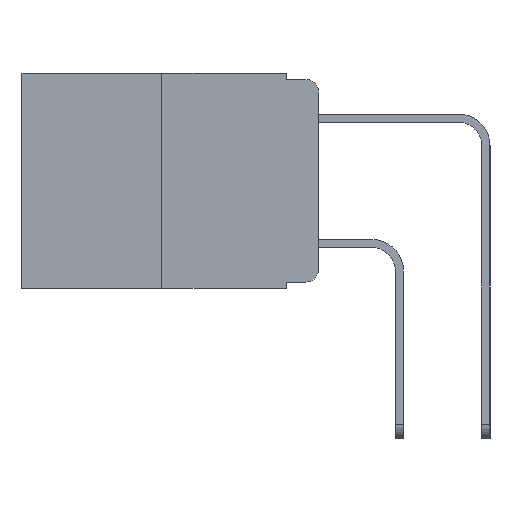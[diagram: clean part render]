
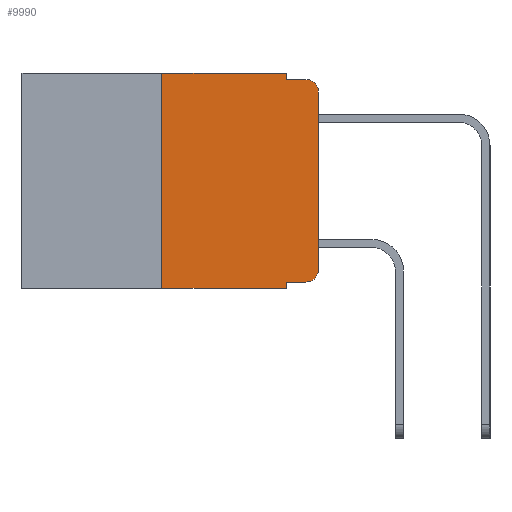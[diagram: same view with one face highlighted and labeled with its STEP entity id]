
A CAD part, left-side view. The second image highlights one B-rep face of the part: STEP entity #9990.
In plain terms, the highlighted planar face has unit normal (-1, 0, 0).
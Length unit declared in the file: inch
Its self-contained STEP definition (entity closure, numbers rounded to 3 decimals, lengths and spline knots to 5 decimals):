
#98 = ORIENTED_EDGE ( 'NONE', *, *, #17553, .T. ) ;
#219 = DIRECTION ( 'NONE',  ( 0., 0., -1. ) ) ;
#268 = VERTEX_POINT ( 'NONE', #16580 ) ;
#549 = CARTESIAN_POINT ( 'NONE',  ( 0., 0.25, -0.343 ) ) ;
#635 = ORIENTED_EDGE ( 'NONE', *, *, #16652, .T. ) ;
#702 = CARTESIAN_POINT ( 'NONE',  ( 0., 0.25, 0. ) ) ;
#779 = CARTESIAN_POINT ( 'NONE',  ( 0., 0.25, 0. ) ) ;
#1356 = DIRECTION ( 'NONE',  ( 0., 0., -1. ) ) ;
#1405 = DIRECTION ( 'NONE',  ( 1., 0., 0. ) ) ;
#2055 = DIRECTION ( 'NONE',  ( -1., 0., 0. ) ) ;
#2135 = ORIENTED_EDGE ( 'NONE', *, *, #11175, .F. ) ;
#2641 = CARTESIAN_POINT ( 'NONE',  ( 0., 0.473, -0.343 ) ) ;
#2648 = LINE ( 'NONE', #13618, #13686 ) ;
#3082 = ORIENTED_EDGE ( 'NONE', *, *, #9319, .T. ) ;
#3471 = DIRECTION ( 'NONE',  ( 0., -1., 0. ) ) ;
#3712 = VERTEX_POINT ( 'NONE', #13400 ) ;
#4144 = CARTESIAN_POINT ( 'NONE',  ( 0., 0.051, -0.343 ) ) ;
#4485 = LINE ( 'NONE', #10110, #15308 ) ;
#4498 = DIRECTION ( 'NONE',  ( 0., -1., 0. ) ) ;
#4771 = ORIENTED_EDGE ( 'NONE', *, *, #13939, .F. ) ;
#5252 = ORIENTED_EDGE ( 'NONE', *, *, #15649, .F. ) ;
#5680 = EDGE_CURVE ( 'NONE', #7753, #17793, #7716, .T. ) ;
#5697 = ORIENTED_EDGE ( 'NONE', *, *, #5680, .T. ) ;
#5949 = VECTOR ( 'NONE', #3471, 39.37008 ) ;
#6074 = AXIS2_PLACEMENT_3D ( 'NONE', #18341, #10202, #1356 ) ;
#6321 = LINE ( 'NONE', #15353, #13356 ) ;
#6624 = VERTEX_POINT ( 'NONE', #16514 ) ;
#6629 = VERTEX_POINT ( 'NONE', #9764 ) ;
#7423 = VECTOR ( 'NONE', #4498, 39.37008 ) ;
#7716 = LINE ( 'NONE', #2641, #18232 ) ;
#7753 = VERTEX_POINT ( 'NONE', #549 ) ;
#8211 = DIRECTION ( 'NONE',  ( 0., 0., 1. ) ) ;
#8399 = VECTOR ( 'NONE', #8211, 39.37008 ) ;
#8627 = ORIENTED_EDGE ( 'NONE', *, *, #12988, .F. ) ;
#8832 = CARTESIAN_POINT ( 'NONE',  ( 0., 0.473, 0. ) ) ;
#9098 = ORIENTED_EDGE ( 'NONE', *, *, #12063, .F. ) ;
#9133 = VERTEX_POINT ( 'NONE', #779 ) ;
#9141 = CARTESIAN_POINT ( 'NONE',  ( 0., 0.051, -0.333 ) ) ;
#9205 = VERTEX_POINT ( 'NONE', #15371 ) ;
#9319 = EDGE_CURVE ( 'NONE', #3712, #6624, #9374, .T. ) ;
#9374 = CIRCLE ( 'NONE', #6074, 0.02 ) ;
#9526 = DIRECTION ( 'NONE',  ( 0., 0., 1. ) ) ;
#9764 = CARTESIAN_POINT ( 'NONE',  ( 0., 0., -0.03 ) ) ;
#9990 = ADVANCED_FACE ( 'NONE', ( #15995 ), #18376, .F. ) ;
#10110 = CARTESIAN_POINT ( 'NONE',  ( 0., 0.051, 0. ) ) ;
#10163 = AXIS2_PLACEMENT_3D ( 'NONE', #10243, #1405, #11618 ) ;
#10202 = DIRECTION ( 'NONE',  ( -1., 0., 0. ) ) ;
#10243 = CARTESIAN_POINT ( 'NONE',  ( 0., 0.473, 0. ) ) ;
#10250 = EDGE_CURVE ( 'NONE', #16461, #3712, #12535, .T. ) ;
#10392 = CARTESIAN_POINT ( 'NONE',  ( 0., 0.051, 0. ) ) ;
#10850 = CARTESIAN_POINT ( 'NONE',  ( 0., 0.02, -0.03 ) ) ;
#10876 = LINE ( 'NONE', #16086, #14536 ) ;
#11164 = LINE ( 'NONE', #8832, #7423 ) ;
#11175 = EDGE_CURVE ( 'NONE', #16461, #17793, #10876, .T. ) ;
#11291 = EDGE_LOOP ( 'NONE', ( #98, #635, #4771, #8627, #5252, #9098, #5697, #2135, #13634, #3082 ) ) ;
#11362 = DIRECTION ( 'NONE',  ( 0., -1., 0. ) ) ;
#11500 = DIRECTION ( 'NONE',  ( 0., 0., -1. ) ) ;
#11618 = DIRECTION ( 'NONE',  ( 0., 0., -1. ) ) ;
#11768 = VERTEX_POINT ( 'NONE', #10392 ) ;
#12063 = EDGE_CURVE ( 'NONE', #7753, #9133, #12510, .T. ) ;
#12068 = CARTESIAN_POINT ( 'NONE',  ( 0., 0.051, -0.333 ) ) ;
#12188 = DIRECTION ( 'NONE',  ( 0., 0., -1. ) ) ;
#12510 = LINE ( 'NONE', #702, #8399 ) ;
#12535 = LINE ( 'NONE', #12068, #5949 ) ;
#12813 = CIRCLE ( 'NONE', #16359, 0.02 ) ;
#12988 = EDGE_CURVE ( 'NONE', #11768, #268, #4485, .T. ) ;
#13356 = VECTOR ( 'NONE', #16740, 39.37008 ) ;
#13400 = CARTESIAN_POINT ( 'NONE',  ( 0., 0.02, -0.333 ) ) ;
#13618 = CARTESIAN_POINT ( 'NONE',  ( 0., 0., 0. ) ) ;
#13634 = ORIENTED_EDGE ( 'NONE', *, *, #10250, .T. ) ;
#13686 = VECTOR ( 'NONE', #9526, 39.37008 ) ;
#13939 = EDGE_CURVE ( 'NONE', #268, #9205, #6321, .T. ) ;
#14536 = VECTOR ( 'NONE', #219, 39.37008 ) ;
#15308 = VECTOR ( 'NONE', #11500, 39.37008 ) ;
#15353 = CARTESIAN_POINT ( 'NONE',  ( 0., 0.051, -0.01 ) ) ;
#15371 = CARTESIAN_POINT ( 'NONE',  ( 0., 0.02, -0.01 ) ) ;
#15649 = EDGE_CURVE ( 'NONE', #9133, #11768, #11164, .T. ) ;
#15995 = FACE_OUTER_BOUND ( 'NONE', #11291, .T. ) ;
#16086 = CARTESIAN_POINT ( 'NONE',  ( 0., 0.051, 0. ) ) ;
#16359 = AXIS2_PLACEMENT_3D ( 'NONE', #10850, #2055, #12188 ) ;
#16461 = VERTEX_POINT ( 'NONE', #9141 ) ;
#16514 = CARTESIAN_POINT ( 'NONE',  ( 0., 0., -0.313 ) ) ;
#16580 = CARTESIAN_POINT ( 'NONE',  ( 0., 0.051, -0.01 ) ) ;
#16652 = EDGE_CURVE ( 'NONE', #6629, #9205, #12813, .T. ) ;
#16740 = DIRECTION ( 'NONE',  ( 0., -1., 0. ) ) ;
#17553 = EDGE_CURVE ( 'NONE', #6624, #6629, #2648, .T. ) ;
#17793 = VERTEX_POINT ( 'NONE', #4144 ) ;
#18232 = VECTOR ( 'NONE', #11362, 39.37008 ) ;
#18341 = CARTESIAN_POINT ( 'NONE',  ( 0., 0.02, -0.313 ) ) ;
#18376 = PLANE ( 'NONE',  #10163 ) ;
